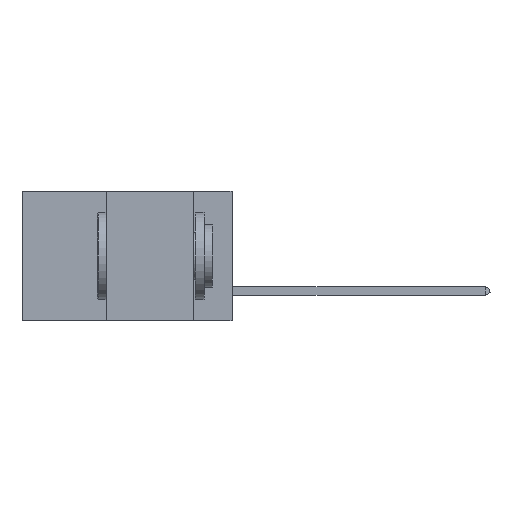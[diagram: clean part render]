
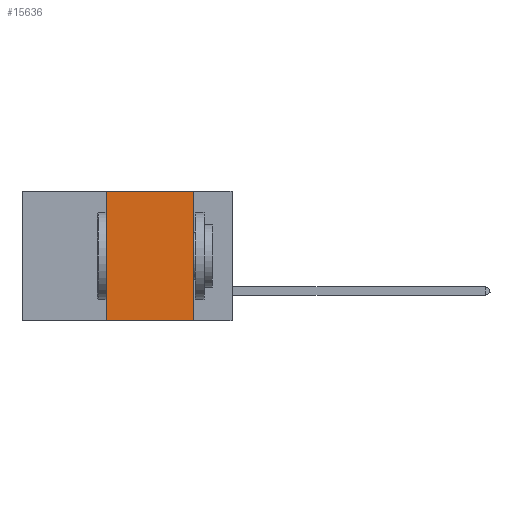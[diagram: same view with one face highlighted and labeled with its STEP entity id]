
A CAD part, left-side view. The second image highlights one B-rep face of the part: STEP entity #15636.
In plain terms, the highlighted planar face has unit normal (-1, 0, 0).
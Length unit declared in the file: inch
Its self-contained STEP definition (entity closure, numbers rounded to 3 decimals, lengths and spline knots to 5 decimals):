
#9 = EDGE_LOOP ( 'NONE', ( #8670, #7545, #12879, #15948 ) ) ;
#633 = DIRECTION ( 'NONE',  ( 0., -1., 0. ) ) ;
#915 = CARTESIAN_POINT ( 'NONE',  ( 0., 0.36, 0. ) ) ;
#1311 = CARTESIAN_POINT ( 'NONE',  ( 0., 0.36, 0. ) ) ;
#1756 = AXIS2_PLACEMENT_3D ( 'NONE', #9148, #4804, #10286 ) ;
#1815 = CARTESIAN_POINT ( 'NONE',  ( 0., 0.11, -0.37 ) ) ;
#2420 = EDGE_CURVE ( 'NONE', #13777, #14929, #7874, .T. ) ;
#3198 = EDGE_CURVE ( 'NONE', #14929, #16516, #16791, .T. ) ;
#4804 = DIRECTION ( 'NONE',  ( 1., 0., 0. ) ) ;
#5009 = VECTOR ( 'NONE', #8391, 39.37008 ) ;
#5198 = VECTOR ( 'NONE', #633, 39.37008 ) ;
#5429 = CARTESIAN_POINT ( 'NONE',  ( 0., 0.11, 0. ) ) ;
#7545 = ORIENTED_EDGE ( 'NONE', *, *, #3198, .F. ) ;
#7750 = VERTEX_POINT ( 'NONE', #1815 ) ;
#7754 = PLANE ( 'NONE',  #1756 ) ;
#7874 = LINE ( 'NONE', #1311, #5009 ) ;
#8391 = DIRECTION ( 'NONE',  ( 0., 0., 1. ) ) ;
#8550 = CARTESIAN_POINT ( 'NONE',  ( 0., 0.36, -0.37 ) ) ;
#8670 = ORIENTED_EDGE ( 'NONE', *, *, #9359, .F. ) ;
#9148 = CARTESIAN_POINT ( 'NONE',  ( 0., 0.6, 0. ) ) ;
#9359 = EDGE_CURVE ( 'NONE', #16516, #7750, #11894, .T. ) ;
#9660 = DIRECTION ( 'NONE',  ( 0., 0., -1. ) ) ;
#10286 = DIRECTION ( 'NONE',  ( 0., 0., -1. ) ) ;
#11614 = CARTESIAN_POINT ( 'NONE',  ( 0., 0.11, 0. ) ) ;
#11632 = EDGE_CURVE ( 'NONE', #13777, #7750, #13448, .T. ) ;
#11665 = VECTOR ( 'NONE', #9660, 39.37008 ) ;
#11894 = LINE ( 'NONE', #5429, #11665 ) ;
#12219 = FACE_OUTER_BOUND ( 'NONE', #9, .T. ) ;
#12879 = ORIENTED_EDGE ( 'NONE', *, *, #2420, .F. ) ;
#13448 = LINE ( 'NONE', #17796, #14551 ) ;
#13627 = DIRECTION ( 'NONE',  ( 0., -1., 0. ) ) ;
#13777 = VERTEX_POINT ( 'NONE', #8550 ) ;
#14551 = VECTOR ( 'NONE', #13627, 39.37008 ) ;
#14929 = VERTEX_POINT ( 'NONE', #915 ) ;
#15636 = ADVANCED_FACE ( 'NONE', ( #12219 ), #7754, .F. ) ;
#15948 = ORIENTED_EDGE ( 'NONE', *, *, #11632, .T. ) ;
#16516 = VERTEX_POINT ( 'NONE', #11614 ) ;
#16791 = LINE ( 'NONE', #17323, #5198 ) ;
#17323 = CARTESIAN_POINT ( 'NONE',  ( 0., 0.6, 0. ) ) ;
#17796 = CARTESIAN_POINT ( 'NONE',  ( 0., 0.6, -0.37 ) ) ;
